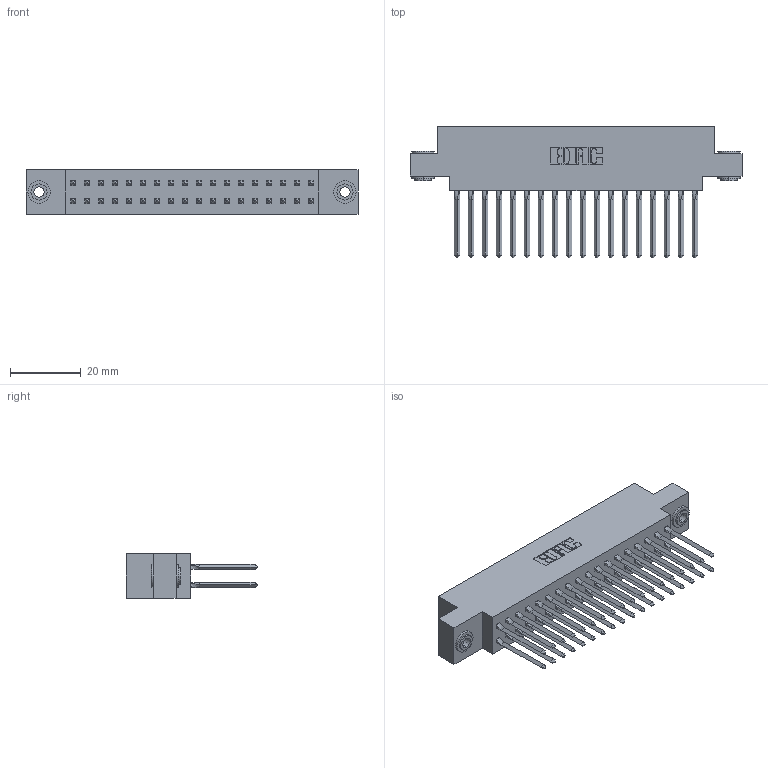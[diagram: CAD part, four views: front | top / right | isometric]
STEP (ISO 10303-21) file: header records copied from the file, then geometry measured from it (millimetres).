
FILE_DESCRIPTION (( 'STEP AP203' ), '1' );
FILE_NAME ('317-036-542-803.STEP', '2020-02-27T22:51:37', ( '' ), ( '' ), 'SwSTEP 2.0', 'SolidWorks 2016', '' );
FILE_SCHEMA (( 'CONFIG_CONTROL_DESIGN' ));
Length unit declared in the file: inch
Products named in the file (4): 317-036-542-803; 317-290-003_542; 317 Part_.156 Dia - TH; 345-250-002_345-250-002-102
Assembly tree (39 placements, depth 2):
  317-036-542-803
    317 Part_.156 Dia - TH
    317-290-003_542  x36
    345-250-002_345-250-002-102  x2
Bounding box: 94.03 x 37.34 x 12.7 mm (x, y, z)
Volume: 14658.2 mm3; surface area: 19829.7 mm2
Topology: 39 solids, 39 shells, 2192 faces, 6111 edges, 3902 vertices
Faces by surface type: plane 1724, cylinder 316, bspline 144, cone 8
Entity records: 29034 total; most frequent: CARTESIAN_POINT 5280, ORIENTED_EDGE 4936, DIRECTION 4234, EDGE_CURVE 2468, LINE 2274, VECTOR 2274, VERTEX_POINT 1638, AXIS2_PLACEMENT_3D 980
